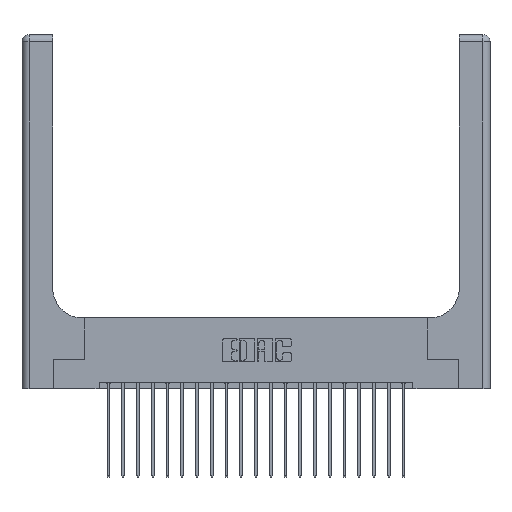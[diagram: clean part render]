
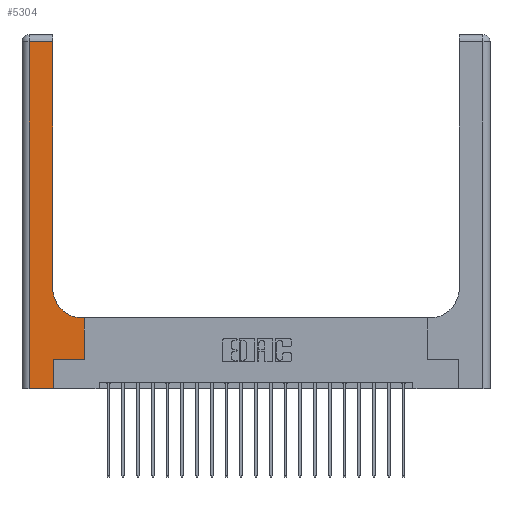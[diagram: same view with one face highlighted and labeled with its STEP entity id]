
A CAD part, top view. The second image highlights one B-rep face of the part: STEP entity #5304.
In plain terms, the highlighted planar face has unit normal (0, 0, 1).
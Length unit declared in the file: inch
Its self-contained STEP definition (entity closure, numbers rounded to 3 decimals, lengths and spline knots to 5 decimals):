
#510 = CARTESIAN_POINT ( 'NONE',  ( 0.06, 3., 0.37 ) ) ;
#786 = CARTESIAN_POINT ( 'NONE',  ( 0.26, 2.94, 0.37 ) ) ;
#1292 = LINE ( 'NONE', #6583, #8247 ) ;
#1738 = EDGE_CURVE ( 'NONE', #5466, #21103, #12207, .T. ) ;
#2099 = CARTESIAN_POINT ( 'NONE',  ( 0., 2.94, 0.37 ) ) ;
#2522 = ORIENTED_EDGE ( 'NONE', *, *, #15604, .T. ) ;
#2525 = LINE ( 'NONE', #9392, #5070 ) ;
#2989 = DIRECTION ( 'NONE',  ( 1., 0., 0. ) ) ;
#3805 = LINE ( 'NONE', #2099, #14168 ) ;
#3829 = ORIENTED_EDGE ( 'NONE', *, *, #21998, .T. ) ;
#4125 = DIRECTION ( 'NONE',  ( -1., 0., 0. ) ) ;
#4313 = CARTESIAN_POINT ( 'NONE',  ( 0.06, 2.94, 0.37 ) ) ;
#4744 = VECTOR ( 'NONE', #2989, 39.37008 ) ;
#5070 = VECTOR ( 'NONE', #10743, 39.37008 ) ;
#5204 = CARTESIAN_POINT ( 'NONE',  ( 0.528, 0.6, 0.37 ) ) ;
#5285 = LINE ( 'NONE', #16965, #15745 ) ;
#5304 = ADVANCED_FACE ( 'NONE', ( #12086 ), #18902, .F. ) ;
#5466 = VERTEX_POINT ( 'NONE', #4313 ) ;
#5564 = CARTESIAN_POINT ( 'NONE',  ( 0., 3., 0.37 ) ) ;
#5618 = ORIENTED_EDGE ( 'NONE', *, *, #14331, .T. ) ;
#5823 = CARTESIAN_POINT ( 'NONE',  ( 0.265, 0.25, 0.37 ) ) ;
#6026 = CARTESIAN_POINT ( 'NONE',  ( 0.528, 0.25, 0.37 ) ) ;
#6120 = EDGE_CURVE ( 'NONE', #21252, #8413, #5285, .T. ) ;
#6428 = AXIS2_PLACEMENT_3D ( 'NONE', #13606, #8245, #14947 ) ;
#6583 = CARTESIAN_POINT ( 'NONE',  ( 0.528, 0.25, 0.37 ) ) ;
#6819 = DIRECTION ( 'NONE',  ( 0., 1., 0. ) ) ;
#7378 = EDGE_LOOP ( 'NONE', ( #14130, #3829, #21674, #2522, #9674, #10731, #9653, #5618, #15395 ) ) ;
#8245 = DIRECTION ( 'NONE',  ( 0., 0., -1. ) ) ;
#8247 = VECTOR ( 'NONE', #13405, 39.37008 ) ;
#8399 = LINE ( 'NONE', #22156, #14239 ) ;
#8413 = VERTEX_POINT ( 'NONE', #786 ) ;
#9348 = CARTESIAN_POINT ( 'NONE',  ( 0.06, 0., 0.37 ) ) ;
#9392 = CARTESIAN_POINT ( 'NONE',  ( 0.26, 0.6, 0.37 ) ) ;
#9653 = ORIENTED_EDGE ( 'NONE', *, *, #11266, .T. ) ;
#9672 = EDGE_CURVE ( 'NONE', #15962, #17957, #8399, .T. ) ;
#9674 = ORIENTED_EDGE ( 'NONE', *, *, #9672, .T. ) ;
#10041 = EDGE_CURVE ( 'NONE', #14919, #21252, #16806, .T. ) ;
#10348 = DIRECTION ( 'NONE',  ( 0., 1., 0. ) ) ;
#10401 = DIRECTION ( 'NONE',  ( -1., 0., 0. ) ) ;
#10717 = CARTESIAN_POINT ( 'NONE',  ( 0.265, 0.25, 0.37 ) ) ;
#10731 = ORIENTED_EDGE ( 'NONE', *, *, #15844, .T. ) ;
#10743 = DIRECTION ( 'NONE',  ( -1., 0., 0. ) ) ;
#11266 = EDGE_CURVE ( 'NONE', #18489, #17280, #1292, .T. ) ;
#11271 = CARTESIAN_POINT ( 'NONE',  ( 0.265, 0., 0.37 ) ) ;
#11407 = CARTESIAN_POINT ( 'NONE',  ( 0., 0., 0.37 ) ) ;
#12086 = FACE_OUTER_BOUND ( 'NONE', #7378, .T. ) ;
#12207 = LINE ( 'NONE', #510, #17992 ) ;
#12993 = VECTOR ( 'NONE', #14259, 39.37008 ) ;
#13084 = LINE ( 'NONE', #11407, #4744 ) ;
#13405 = DIRECTION ( 'NONE',  ( 0., 1., 0. ) ) ;
#13606 = CARTESIAN_POINT ( 'NONE',  ( 0.51, 0.85, 0.37 ) ) ;
#14130 = ORIENTED_EDGE ( 'NONE', *, *, #6120, .T. ) ;
#14168 = VECTOR ( 'NONE', #4125, 39.37008 ) ;
#14239 = VECTOR ( 'NONE', #6819, 39.37008 ) ;
#14259 = DIRECTION ( 'NONE',  ( 1., 0., 0. ) ) ;
#14331 = EDGE_CURVE ( 'NONE', #17280, #14919, #2525, .T. ) ;
#14919 = VERTEX_POINT ( 'NONE', #20317 ) ;
#14947 = DIRECTION ( 'NONE',  ( 1., 0., 0. ) ) ;
#15395 = ORIENTED_EDGE ( 'NONE', *, *, #10041, .T. ) ;
#15604 = EDGE_CURVE ( 'NONE', #21103, #15962, #13084, .T. ) ;
#15745 = VECTOR ( 'NONE', #10348, 39.37008 ) ;
#15844 = EDGE_CURVE ( 'NONE', #17957, #18489, #19326, .T. ) ;
#15962 = VERTEX_POINT ( 'NONE', #11271 ) ;
#16806 = CIRCLE ( 'NONE', #6428, 0.25 ) ;
#16965 = CARTESIAN_POINT ( 'NONE',  ( 0.26, 3., 0.37 ) ) ;
#17280 = VERTEX_POINT ( 'NONE', #5204 ) ;
#17957 = VERTEX_POINT ( 'NONE', #5823 ) ;
#17992 = VECTOR ( 'NONE', #19787, 39.37008 ) ;
#18489 = VERTEX_POINT ( 'NONE', #6026 ) ;
#18853 = AXIS2_PLACEMENT_3D ( 'NONE', #5564, #19125, #10401 ) ;
#18902 = PLANE ( 'NONE',  #18853 ) ;
#19125 = DIRECTION ( 'NONE',  ( 0., 0., -1. ) ) ;
#19326 = LINE ( 'NONE', #10717, #12993 ) ;
#19787 = DIRECTION ( 'NONE',  ( 0., -1., 0. ) ) ;
#20193 = CARTESIAN_POINT ( 'NONE',  ( 0.26, 0.85, 0.37 ) ) ;
#20317 = CARTESIAN_POINT ( 'NONE',  ( 0.51, 0.6, 0.37 ) ) ;
#21103 = VERTEX_POINT ( 'NONE', #9348 ) ;
#21252 = VERTEX_POINT ( 'NONE', #20193 ) ;
#21674 = ORIENTED_EDGE ( 'NONE', *, *, #1738, .T. ) ;
#21998 = EDGE_CURVE ( 'NONE', #8413, #5466, #3805, .T. ) ;
#22156 = CARTESIAN_POINT ( 'NONE',  ( 0.265, 0., 0.37 ) ) ;
